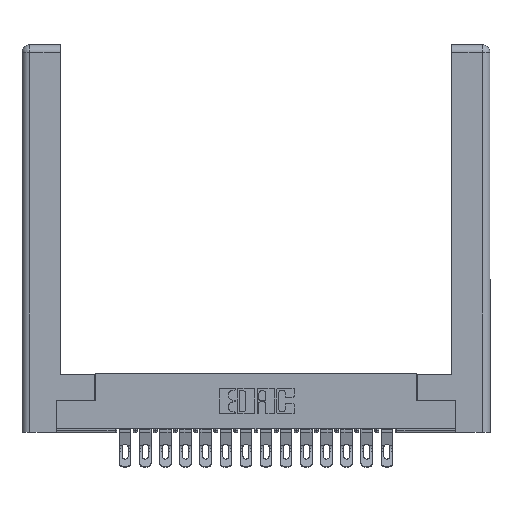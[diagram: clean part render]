
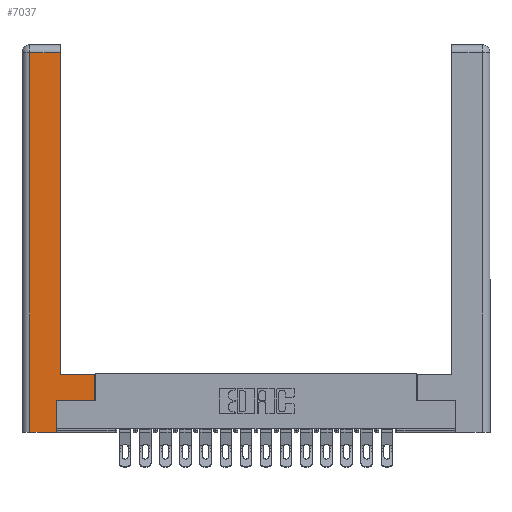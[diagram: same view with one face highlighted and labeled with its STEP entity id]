
A CAD part, top view. The second image highlights one B-rep face of the part: STEP entity #7037.
In plain terms, the highlighted planar face has unit normal (0, 0, 1).
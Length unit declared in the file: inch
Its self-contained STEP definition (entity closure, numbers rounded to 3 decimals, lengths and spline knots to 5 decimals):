
#253 = VERTEX_POINT ( 'NONE', #12464 ) ;
#364 = EDGE_CURVE ( 'NONE', #14258, #4247, #2570, .T. ) ;
#365 = LINE ( 'NONE', #9096, #12508 ) ;
#615 = DIRECTION ( 'NONE',  ( 0., 1., 0. ) ) ;
#928 = DIRECTION ( 'NONE',  ( 0., 1., 0. ) ) ;
#1081 = CARTESIAN_POINT ( 'NONE',  ( 0.295, 2.94, 0. ) ) ;
#1133 = VECTOR ( 'NONE', #5754, 39.37008 ) ;
#1150 = VERTEX_POINT ( 'NONE', #8901 ) ;
#1583 = CARTESIAN_POINT ( 'NONE',  ( 0.0615, 2.94, 0. ) ) ;
#1902 = DIRECTION ( 'NONE',  ( 0., -1., 0. ) ) ;
#2364 = VECTOR ( 'NONE', #18564, 39.37008 ) ;
#2440 = EDGE_CURVE ( 'NONE', #10151, #11388, #5144, .T. ) ;
#2570 = LINE ( 'NONE', #19505, #19958 ) ;
#2788 = VECTOR ( 'NONE', #615, 39.37008 ) ;
#2895 = VERTEX_POINT ( 'NONE', #9022 ) ;
#2981 = EDGE_CURVE ( 'NONE', #2895, #14258, #6725, .T. ) ;
#3419 = ORIENTED_EDGE ( 'NONE', *, *, #364, .T. ) ;
#3495 = CARTESIAN_POINT ( 'NONE',  ( 0.295, 0.45, 0. ) ) ;
#3519 = LINE ( 'NONE', #5129, #15880 ) ;
#4247 = VERTEX_POINT ( 'NONE', #1081 ) ;
#4282 = CARTESIAN_POINT ( 'NONE',  ( 0.295, 0.45, 0. ) ) ;
#5129 = CARTESIAN_POINT ( 'NONE',  ( 0.0615, 2.94, 0. ) ) ;
#5144 = LINE ( 'NONE', #13468, #10447 ) ;
#5232 = EDGE_CURVE ( 'NONE', #12449, #253, #365, .T. ) ;
#5301 = ORIENTED_EDGE ( 'NONE', *, *, #17278, .T. ) ;
#5333 = LINE ( 'NONE', #5447, #9303 ) ;
#5447 = CARTESIAN_POINT ( 'NONE',  ( 0.265, 0., 0. ) ) ;
#5744 = ORIENTED_EDGE ( 'NONE', *, *, #2440, .T. ) ;
#5754 = DIRECTION ( 'NONE',  ( -1., 0., 0. ) ) ;
#5936 = PLANE ( 'NONE',  #15142 ) ;
#6345 = ORIENTED_EDGE ( 'NONE', *, *, #5232, .T. ) ;
#6712 = EDGE_CURVE ( 'NONE', #11388, #12449, #5333, .T. ) ;
#6725 = LINE ( 'NONE', #4282, #1133 ) ;
#7037 = ADVANCED_FACE ( 'NONE', ( #19761 ), #5936, .F. ) ;
#7382 = CARTESIAN_POINT ( 'NONE',  ( 0.265, 0., 0. ) ) ;
#8901 = CARTESIAN_POINT ( 'NONE',  ( 0.565, 0.245, 0. ) ) ;
#9022 = CARTESIAN_POINT ( 'NONE',  ( 0.565, 0.45, 0. ) ) ;
#9096 = CARTESIAN_POINT ( 'NONE',  ( 0.265, 0.245, 0. ) ) ;
#9303 = VECTOR ( 'NONE', #20908, 39.37008 ) ;
#10151 = VERTEX_POINT ( 'NONE', #1583 ) ;
#10444 = ORIENTED_EDGE ( 'NONE', *, *, #2981, .T. ) ;
#10447 = VECTOR ( 'NONE', #1902, 39.37008 ) ;
#10650 = EDGE_CURVE ( 'NONE', #1150, #2895, #17812, .T. ) ;
#10844 = EDGE_LOOP ( 'NONE', ( #3419, #18361, #5744, #19474, #6345, #5301, #12093, #10444 ) ) ;
#10980 = CARTESIAN_POINT ( 'NONE',  ( 0.565, 0.45, 0. ) ) ;
#11388 = VERTEX_POINT ( 'NONE', #17861 ) ;
#12093 = ORIENTED_EDGE ( 'NONE', *, *, #10650, .T. ) ;
#12449 = VERTEX_POINT ( 'NONE', #7382 ) ;
#12464 = CARTESIAN_POINT ( 'NONE',  ( 0.265, 0.245, 0. ) ) ;
#12508 = VECTOR ( 'NONE', #17679, 39.37008 ) ;
#12698 = CARTESIAN_POINT ( 'NONE',  ( 0., 0., 0. ) ) ;
#12831 = DIRECTION ( 'NONE',  ( 0., 0., -1. ) ) ;
#13468 = CARTESIAN_POINT ( 'NONE',  ( 0.0615, 0., 0. ) ) ;
#14258 = VERTEX_POINT ( 'NONE', #3495 ) ;
#14608 = DIRECTION ( 'NONE',  ( -1., 0., 0. ) ) ;
#15142 = AXIS2_PLACEMENT_3D ( 'NONE', #12698, #12831, #14608 ) ;
#15880 = VECTOR ( 'NONE', #17875, 39.37008 ) ;
#16480 = CARTESIAN_POINT ( 'NONE',  ( 0.565, 0.245, 0. ) ) ;
#17278 = EDGE_CURVE ( 'NONE', #253, #1150, #17394, .T. ) ;
#17394 = LINE ( 'NONE', #16480, #2364 ) ;
#17679 = DIRECTION ( 'NONE',  ( 0., 1., 0. ) ) ;
#17812 = LINE ( 'NONE', #10980, #2788 ) ;
#17861 = CARTESIAN_POINT ( 'NONE',  ( 0.0615, 0., 0. ) ) ;
#17875 = DIRECTION ( 'NONE',  ( -1., 0., 0. ) ) ;
#18361 = ORIENTED_EDGE ( 'NONE', *, *, #19772, .T. ) ;
#18564 = DIRECTION ( 'NONE',  ( 1., 0., 0. ) ) ;
#19474 = ORIENTED_EDGE ( 'NONE', *, *, #6712, .T. ) ;
#19505 = CARTESIAN_POINT ( 'NONE',  ( 0.295, 3., 0. ) ) ;
#19761 = FACE_OUTER_BOUND ( 'NONE', #10844, .T. ) ;
#19772 = EDGE_CURVE ( 'NONE', #4247, #10151, #3519, .T. ) ;
#19958 = VECTOR ( 'NONE', #928, 39.37008 ) ;
#20908 = DIRECTION ( 'NONE',  ( 1., 0., 0. ) ) ;
